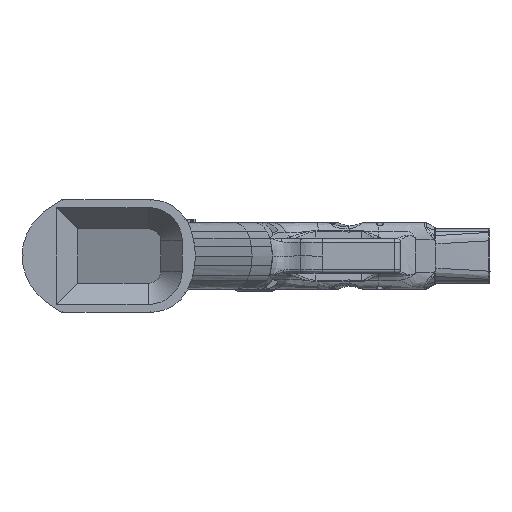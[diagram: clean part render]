
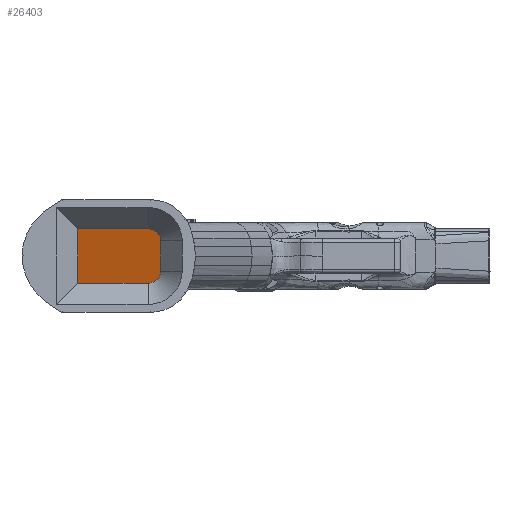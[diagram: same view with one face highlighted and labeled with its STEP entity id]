
A CAD part, front view. The second image highlights one B-rep face of the part: STEP entity #26403.
In plain terms, the highlighted planar face has unit normal (0.951, -0.309, 0).
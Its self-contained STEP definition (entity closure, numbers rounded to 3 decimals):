
#521 = LINE ( 'NONE', #54018, #38933 ) ;
#1127 = DIRECTION ( 'NONE',  ( 0.309, 0.951, 0. ) ) ;
#1316 = DIRECTION ( 'NONE',  ( 0., 0., -1. ) ) ;
#2302 = EDGE_CURVE ( 'NONE', #21067, #41902, #521, .T. ) ;
#7913 = ORIENTED_EDGE ( 'NONE', *, *, #17899, .F. ) ;
#8823 = CARTESIAN_POINT ( 'NONE',  ( 32.169, -5.875, -10.375 ) ) ;
#9557 = CARTESIAN_POINT ( 'NONE',  ( 32.169, -5.875, -11.75 ) ) ;
#11938 = EDGE_CURVE ( 'NONE', #46708, #41902, #24985, .T. ) ;
#12082 = PLANE ( 'NONE',  #53460 ) ;
#12268 = DIRECTION ( 'NONE',  ( 0., 0., -1. ) ) ;
#13911 = EDGE_CURVE ( 'NONE', #22887, #51749, #27758, .T. ) ;
#14786 = DIRECTION ( 'NONE',  ( -0.309, -0.951, 0. ) ) ;
#15726 = CARTESIAN_POINT ( 'NONE',  ( 33.591, -1.5, -10.375 ) ) ;
#16904 = DIRECTION ( 'NONE',  ( -0.951, 0.309, 0. ) ) ;
#17546 = DIRECTION ( 'NONE',  ( -0.309, -0.951, 0. ) ) ;
#17720 = LINE ( 'NONE', #28021, #28480 ) ;
#17899 = EDGE_CURVE ( 'NONE', #51749, #46708, #17720, .T. ) ;
#18981 = CARTESIAN_POINT ( 'NONE',  ( 2.312, -97.765, -10.375 ) ) ;
#19938 = LINE ( 'NONE', #18981, #23463 ) ;
#20159 = LINE ( 'NONE', #9557, #30326 ) ;
#21014 = EDGE_CURVE ( 'NONE', #21067, #54173, #19938, .T. ) ;
#21067 = VERTEX_POINT ( 'NONE', #15726 ) ;
#21412 = ORIENTED_EDGE ( 'NONE', *, *, #21014, .F. ) ;
#22887 = VERTEX_POINT ( 'NONE', #42420 ) ;
#22912 = CARTESIAN_POINT ( 'NONE',  ( 2.312, -97.765, 11.75 ) ) ;
#23463 = VECTOR ( 'NONE', #14786, 1000. ) ;
#24864 = LINE ( 'NONE', #40627, #25995 ) ;
#24985 = LINE ( 'NONE', #39496, #57665 ) ;
#25995 = VECTOR ( 'NONE', #1316, 1000. ) ;
#26403 = ADVANCED_FACE ( 'NONE', ( #32681 ), #12082, .F. ) ;
#27758 = LINE ( 'NONE', #22912, #47685 ) ;
#28021 = CARTESIAN_POINT ( 'NONE',  ( 30.049, -12.4, -11.75 ) ) ;
#28480 = VECTOR ( 'NONE', #12268, 1000. ) ;
#29842 = DIRECTION ( 'NONE',  ( 0., 0., 1. ) ) ;
#30326 = VECTOR ( 'NONE', #34340, 1000. ) ;
#31320 = ORIENTED_EDGE ( 'NONE', *, *, #11938, .F. ) ;
#32681 = FACE_OUTER_BOUND ( 'NONE', #39479, .T. ) ;
#33060 = LINE ( 'NONE', #63033, #51950 ) ;
#33480 = CARTESIAN_POINT ( 'NONE',  ( -22.8, -175.052, -11.75 ) ) ;
#34340 = DIRECTION ( 'NONE',  ( -0.309, -0.951, 0. ) ) ;
#35006 = ORIENTED_EDGE ( 'NONE', *, *, #55087, .F. ) ;
#36125 = CARTESIAN_POINT ( 'NONE',  ( 30.049, -12.4, 11.75 ) ) ;
#37455 = ORIENTED_EDGE ( 'NONE', *, *, #59693, .F. ) ;
#38933 = VECTOR ( 'NONE', #29842, 1000. ) ;
#39479 = EDGE_LOOP ( 'NONE', ( #47185, #55231, #35006, #37455, #21412, #51194, #31320, #7913 ) ) ;
#39496 = CARTESIAN_POINT ( 'NONE',  ( 2.312, -97.765, 4.75 ) ) ;
#40243 = VERTEX_POINT ( 'NONE', #33480 ) ;
#40609 = CARTESIAN_POINT ( 'NONE',  ( 32.169, -5.875, -11.75 ) ) ;
#40627 = CARTESIAN_POINT ( 'NONE',  ( -22.8, -175.052, -11.75 ) ) ;
#41902 = VERTEX_POINT ( 'NONE', #50090 ) ;
#42420 = CARTESIAN_POINT ( 'NONE',  ( -22.8, -175.052, 11.75 ) ) ;
#46245 = CARTESIAN_POINT ( 'NONE',  ( 2.312, -97.765, -11.75 ) ) ;
#46708 = VERTEX_POINT ( 'NONE', #51473 ) ;
#47185 = ORIENTED_EDGE ( 'NONE', *, *, #13911, .F. ) ;
#47685 = VECTOR ( 'NONE', #47730, 1000. ) ;
#47730 = DIRECTION ( 'NONE',  ( 0.309, 0.951, 0. ) ) ;
#48212 = DIRECTION ( 'NONE',  ( 0., 0., -1. ) ) ;
#49497 = EDGE_CURVE ( 'NONE', #22887, #40243, #24864, .T. ) ;
#50090 = CARTESIAN_POINT ( 'NONE',  ( 33.591, -1.5, 4.75 ) ) ;
#51194 = ORIENTED_EDGE ( 'NONE', *, *, #2302, .T. ) ;
#51473 = CARTESIAN_POINT ( 'NONE',  ( 30.049, -12.4, 4.75 ) ) ;
#51749 = VERTEX_POINT ( 'NONE', #36125 ) ;
#51950 = VECTOR ( 'NONE', #48212, 1000. ) ;
#53460 = AXIS2_PLACEMENT_3D ( 'NONE', #46245, #16904, #17546 ) ;
#54018 = CARTESIAN_POINT ( 'NONE',  ( 33.591, -1.5, 0. ) ) ;
#54173 = VERTEX_POINT ( 'NONE', #8823 ) ;
#55087 = EDGE_CURVE ( 'NONE', #55342, #40243, #20159, .T. ) ;
#55231 = ORIENTED_EDGE ( 'NONE', *, *, #49497, .T. ) ;
#55342 = VERTEX_POINT ( 'NONE', #40609 ) ;
#57665 = VECTOR ( 'NONE', #1127, 1000. ) ;
#59693 = EDGE_CURVE ( 'NONE', #54173, #55342, #33060, .T. ) ;
#63033 = CARTESIAN_POINT ( 'NONE',  ( 32.169, -5.875, -11.75 ) ) ;
